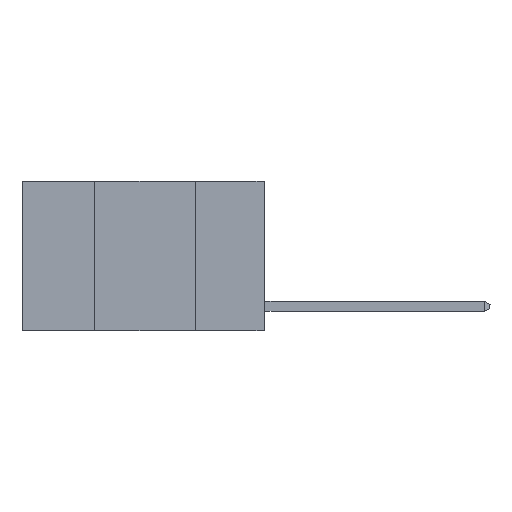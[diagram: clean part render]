
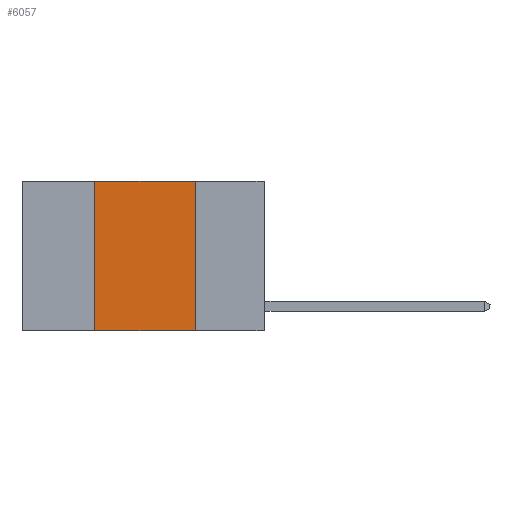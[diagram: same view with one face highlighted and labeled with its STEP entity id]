
A CAD part, left-side view. The second image highlights one B-rep face of the part: STEP entity #6057.
In plain terms, the highlighted planar face has unit normal (-1, 0, 0).
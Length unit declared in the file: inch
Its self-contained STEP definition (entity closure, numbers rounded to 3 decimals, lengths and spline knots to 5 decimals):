
#435 = ORIENTED_EDGE ( 'NONE', *, *, #5085, .T. ) ;
#438 = ORIENTED_EDGE ( 'NONE', *, *, #13179, .F. ) ;
#803 = CARTESIAN_POINT ( 'NONE',  ( 0., 0.6, 0. ) ) ;
#1584 = VECTOR ( 'NONE', #5027, 39.37008 ) ;
#2038 = VECTOR ( 'NONE', #16932, 39.37008 ) ;
#2130 = PLANE ( 'NONE',  #6145 ) ;
#2369 = ORIENTED_EDGE ( 'NONE', *, *, #6595, .F. ) ;
#3474 = VERTEX_POINT ( 'NONE', #4558 ) ;
#3562 = LINE ( 'NONE', #13300, #3980 ) ;
#3980 = VECTOR ( 'NONE', #5380, 39.37008 ) ;
#4362 = VECTOR ( 'NONE', #4497, 39.37008 ) ;
#4497 = DIRECTION ( 'NONE',  ( 0., -1., 0. ) ) ;
#4558 = CARTESIAN_POINT ( 'NONE',  ( 0., 0.42, -0.37 ) ) ;
#5027 = DIRECTION ( 'NONE',  ( 0., 0., -1. ) ) ;
#5085 = EDGE_CURVE ( 'NONE', #3474, #5676, #3562, .T. ) ;
#5380 = DIRECTION ( 'NONE',  ( 0., -1., 0. ) ) ;
#5611 = VERTEX_POINT ( 'NONE', #10496 ) ;
#5676 = VERTEX_POINT ( 'NONE', #11947 ) ;
#6057 = ADVANCED_FACE ( 'NONE', ( #16880 ), #2130, .F. ) ;
#6078 = DIRECTION ( 'NONE',  ( 1., 0., 0. ) ) ;
#6145 = AXIS2_PLACEMENT_3D ( 'NONE', #803, #6078, #15260 ) ;
#6595 = EDGE_CURVE ( 'NONE', #7023, #5611, #11770, .T. ) ;
#7023 = VERTEX_POINT ( 'NONE', #15838 ) ;
#7790 = EDGE_LOOP ( 'NONE', ( #10952, #2369, #438, #435 ) ) ;
#8543 = LINE ( 'NONE', #14207, #1584 ) ;
#10496 = CARTESIAN_POINT ( 'NONE',  ( 0., 0.17, 0. ) ) ;
#10952 = ORIENTED_EDGE ( 'NONE', *, *, #14068, .F. ) ;
#11100 = CARTESIAN_POINT ( 'NONE',  ( 0., 0.6, 0. ) ) ;
#11770 = LINE ( 'NONE', #11100, #4362 ) ;
#11947 = CARTESIAN_POINT ( 'NONE',  ( 0., 0.17, -0.37 ) ) ;
#12964 = CARTESIAN_POINT ( 'NONE',  ( 0., 0.42, 0. ) ) ;
#13179 = EDGE_CURVE ( 'NONE', #3474, #7023, #15964, .T. ) ;
#13300 = CARTESIAN_POINT ( 'NONE',  ( 0., 0.6, -0.37 ) ) ;
#14068 = EDGE_CURVE ( 'NONE', #5611, #5676, #8543, .T. ) ;
#14207 = CARTESIAN_POINT ( 'NONE',  ( 0., 0.17, 0. ) ) ;
#15260 = DIRECTION ( 'NONE',  ( 0., 0., -1. ) ) ;
#15838 = CARTESIAN_POINT ( 'NONE',  ( 0., 0.42, 0. ) ) ;
#15964 = LINE ( 'NONE', #12964, #2038 ) ;
#16880 = FACE_OUTER_BOUND ( 'NONE', #7790, .T. ) ;
#16932 = DIRECTION ( 'NONE',  ( 0., 0., 1. ) ) ;
